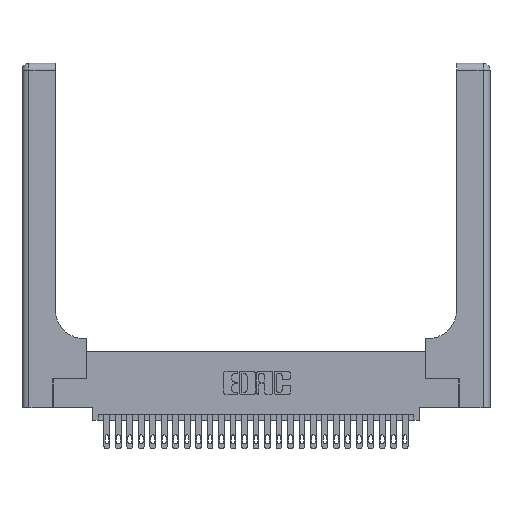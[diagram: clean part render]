
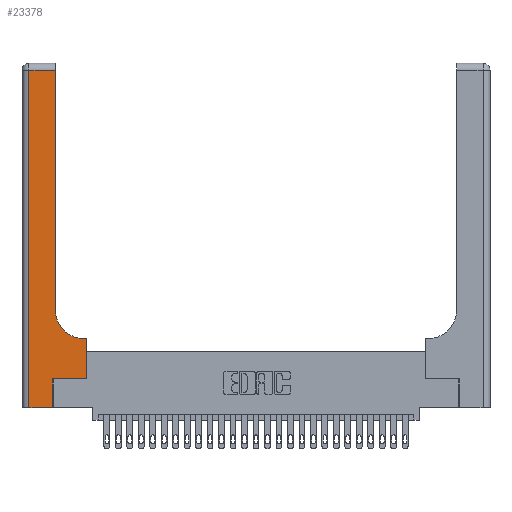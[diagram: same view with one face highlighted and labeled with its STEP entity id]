
A CAD part, top view. The second image highlights one B-rep face of the part: STEP entity #23378.
In plain terms, the highlighted planar face has unit normal (0, 0, 1).
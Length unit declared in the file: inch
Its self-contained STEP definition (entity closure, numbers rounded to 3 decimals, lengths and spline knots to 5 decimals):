
#683 = DIRECTION ( 'NONE',  ( -1., 0., 0. ) ) ;
#736 = ORIENTED_EDGE ( 'NONE', *, *, #15961, .T. ) ;
#1017 = LINE ( 'NONE', #27229, #14095 ) ;
#1052 = LINE ( 'NONE', #17063, #11390 ) ;
#1092 = EDGE_CURVE ( 'NONE', #26727, #21085, #6635, .T. ) ;
#1450 = CARTESIAN_POINT ( 'NONE',  ( 0.2915, 0.85, 0.37 ) ) ;
#1678 = VERTEX_POINT ( 'NONE', #22720 ) ;
#2516 = LINE ( 'NONE', #24136, #25225 ) ;
#3336 = EDGE_CURVE ( 'NONE', #25351, #26727, #1017, .T. ) ;
#3479 = DIRECTION ( 'NONE',  ( 1., 0., 0. ) ) ;
#3566 = ORIENTED_EDGE ( 'NONE', *, *, #21414, .T. ) ;
#4199 = LINE ( 'NONE', #11357, #5561 ) ;
#5394 = ORIENTED_EDGE ( 'NONE', *, *, #7112, .T. ) ;
#5414 = DIRECTION ( 'NONE',  ( -1., 0., 0. ) ) ;
#5561 = VECTOR ( 'NONE', #9809, 39.37008 ) ;
#6307 = VECTOR ( 'NONE', #683, 39.37008 ) ;
#6445 = CARTESIAN_POINT ( 'NONE',  ( 0.269, 0., 0.37 ) ) ;
#6635 = LINE ( 'NONE', #9741, #6307 ) ;
#6699 = VERTEX_POINT ( 'NONE', #24300 ) ;
#7112 = EDGE_CURVE ( 'NONE', #6699, #1678, #4199, .T. ) ;
#7731 = CARTESIAN_POINT ( 'NONE',  ( 0.5415, 0.85, 0.37 ) ) ;
#8907 = CARTESIAN_POINT ( 'NONE',  ( 0.5585, 0.25, 0.37 ) ) ;
#9741 = CARTESIAN_POINT ( 'NONE',  ( 0., 2.94, 0.37 ) ) ;
#9809 = DIRECTION ( 'NONE',  ( 1., 0., 0. ) ) ;
#10334 = CARTESIAN_POINT ( 'NONE',  ( 0.06, 2.94, 0.37 ) ) ;
#11238 = VERTEX_POINT ( 'NONE', #26824 ) ;
#11357 = CARTESIAN_POINT ( 'NONE',  ( 0., 0., 0.37 ) ) ;
#11390 = VECTOR ( 'NONE', #16774, 39.37008 ) ;
#12342 = FACE_OUTER_BOUND ( 'NONE', #15212, .T. ) ;
#12620 = VERTEX_POINT ( 'NONE', #25024 ) ;
#13188 = VECTOR ( 'NONE', #3479, 39.37008 ) ;
#13659 = AXIS2_PLACEMENT_3D ( 'NONE', #7731, #20672, #27132 ) ;
#13932 = CARTESIAN_POINT ( 'NONE',  ( 0.5585, 0.25, 0.37 ) ) ;
#14095 = VECTOR ( 'NONE', #23287, 39.37008 ) ;
#14235 = EDGE_CURVE ( 'NONE', #11238, #26950, #16293, .T. ) ;
#14538 = EDGE_CURVE ( 'NONE', #21085, #6699, #2516, .T. ) ;
#14565 = CARTESIAN_POINT ( 'NONE',  ( 0., 3., 0.37 ) ) ;
#14832 = CIRCLE ( 'NONE', #13659, 0.25 ) ;
#15212 = EDGE_LOOP ( 'NONE', ( #21843, #24996, #26120, #5394, #3566, #16973, #18762, #28364, #736 ) ) ;
#15410 = CARTESIAN_POINT ( 'NONE',  ( 0.2915, 2.94, 0.37 ) ) ;
#15961 = EDGE_CURVE ( 'NONE', #19165, #25351, #14832, .T. ) ;
#16293 = LINE ( 'NONE', #18715, #13188 ) ;
#16774 = DIRECTION ( 'NONE',  ( -1., 0., 0. ) ) ;
#16973 = ORIENTED_EDGE ( 'NONE', *, *, #14235, .T. ) ;
#17063 = CARTESIAN_POINT ( 'NONE',  ( 0.2915, 0.6, 0.37 ) ) ;
#18301 = CARTESIAN_POINT ( 'NONE',  ( 0.5415, 0.6, 0.37 ) ) ;
#18715 = CARTESIAN_POINT ( 'NONE',  ( 0.269, 0.25, 0.37 ) ) ;
#18762 = ORIENTED_EDGE ( 'NONE', *, *, #24981, .T. ) ;
#18846 = PLANE ( 'NONE',  #19433 ) ;
#19165 = VERTEX_POINT ( 'NONE', #18301 ) ;
#19433 = AXIS2_PLACEMENT_3D ( 'NONE', #14565, #23307, #5414 ) ;
#19574 = DIRECTION ( 'NONE',  ( 0., -1., 0. ) ) ;
#20086 = DIRECTION ( 'NONE',  ( 0., 1., 0. ) ) ;
#20089 = VECTOR ( 'NONE', #20086, 39.37008 ) ;
#20672 = DIRECTION ( 'NONE',  ( 0., 0., -1. ) ) ;
#21085 = VERTEX_POINT ( 'NONE', #10334 ) ;
#21414 = EDGE_CURVE ( 'NONE', #1678, #11238, #22352, .T. ) ;
#21843 = ORIENTED_EDGE ( 'NONE', *, *, #3336, .T. ) ;
#21903 = DIRECTION ( 'NONE',  ( 0., 1., 0. ) ) ;
#22352 = LINE ( 'NONE', #6445, #23082 ) ;
#22720 = CARTESIAN_POINT ( 'NONE',  ( 0.269, 0., 0.37 ) ) ;
#23082 = VECTOR ( 'NONE', #21903, 39.37008 ) ;
#23287 = DIRECTION ( 'NONE',  ( 0., 1., 0. ) ) ;
#23307 = DIRECTION ( 'NONE',  ( 0., 0., -1. ) ) ;
#23378 = ADVANCED_FACE ( 'NONE', ( #12342 ), #18846, .F. ) ;
#24136 = CARTESIAN_POINT ( 'NONE',  ( 0.06, 3., 0.37 ) ) ;
#24300 = CARTESIAN_POINT ( 'NONE',  ( 0.06, 0., 0.37 ) ) ;
#24624 = LINE ( 'NONE', #8907, #20089 ) ;
#24981 = EDGE_CURVE ( 'NONE', #26950, #12620, #24624, .T. ) ;
#24996 = ORIENTED_EDGE ( 'NONE', *, *, #1092, .T. ) ;
#25024 = CARTESIAN_POINT ( 'NONE',  ( 0.5585, 0.6, 0.37 ) ) ;
#25225 = VECTOR ( 'NONE', #19574, 39.37008 ) ;
#25351 = VERTEX_POINT ( 'NONE', #1450 ) ;
#26120 = ORIENTED_EDGE ( 'NONE', *, *, #14538, .T. ) ;
#26727 = VERTEX_POINT ( 'NONE', #15410 ) ;
#26824 = CARTESIAN_POINT ( 'NONE',  ( 0.269, 0.25, 0.37 ) ) ;
#26950 = VERTEX_POINT ( 'NONE', #13932 ) ;
#27132 = DIRECTION ( 'NONE',  ( 1., 0., 0. ) ) ;
#27229 = CARTESIAN_POINT ( 'NONE',  ( 0.2915, 3., 0.37 ) ) ;
#27640 = EDGE_CURVE ( 'NONE', #12620, #19165, #1052, .T. ) ;
#28364 = ORIENTED_EDGE ( 'NONE', *, *, #27640, .T. ) ;
